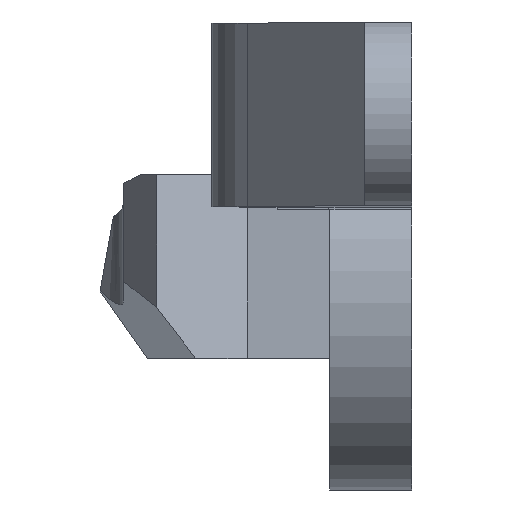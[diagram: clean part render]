
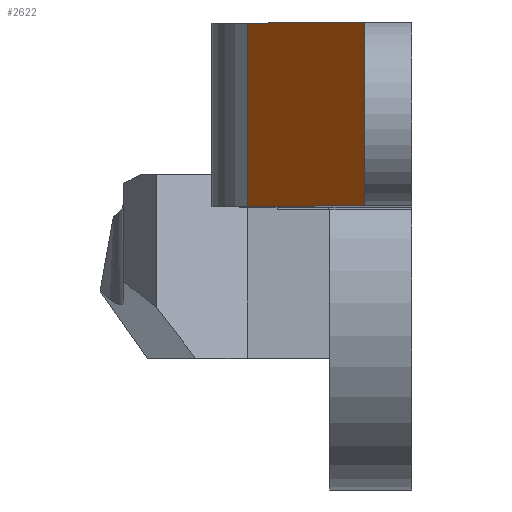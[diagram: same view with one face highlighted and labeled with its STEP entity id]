
A CAD part, top view. The second image highlights one B-rep face of the part: STEP entity #2622.
In plain terms, the highlighted planar face has unit normal (-0.985, 0, 0.174).
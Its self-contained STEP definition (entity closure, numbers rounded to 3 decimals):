
#1336 = PLANE('',#1337);
#1337 = AXIS2_PLACEMENT_3D('',#1338,#1339,#1340);
#1338 = CARTESIAN_POINT('',(-1.916,-1.752,-3.782));
#1339 = DIRECTION('',(0.,1.,0.));
#1340 = DIRECTION('',(0.,0.,1.));
#1388 = PLANE('',#1389);
#1389 = AXIS2_PLACEMENT_3D('',#1390,#1391,#1392);
#1390 = CARTESIAN_POINT('',(9.391,6.048,-3.639));
#1391 = DIRECTION('',(0.,1.,0.));
#1392 = DIRECTION('',(0.,0.,1.));
#2198 = VERTEX_POINT('',#2199);
#2199 = CARTESIAN_POINT('',(0.,6.048,
    -36.438));
#2212 = PLANE('',#2213);
#2213 = AXIS2_PLACEMENT_3D('',#2214,#2215,#2216);
#2214 = CARTESIAN_POINT('',(0.,0.,0.));
#2215 = DIRECTION('',(1.,0.,0.));
#2216 = DIRECTION('',(0.,0.,-1.));
#2223 = EDGE_CURVE('',#2198,#2224,#2226,.T.);
#2224 = VERTEX_POINT('',#2225);
#2225 = CARTESIAN_POINT('',(5.,6.048,-8.082));
#2226 = SURFACE_CURVE('',#2227,(#2231,#2237),.PCURVE_S1.);
#2227 = LINE('',#2228,#2229);
#2228 = CARTESIAN_POINT('',(6.062,6.048,
    -2.06));
#2229 = VECTOR('',#2230,1.);
#2230 = DIRECTION('',(0.174,0.,0.985
    ));
#2231 = PCURVE('',#1388,#2232);
#2232 = DEFINITIONAL_REPRESENTATION('',(#2233),#2236);
#2233 = B_SPLINE_CURVE_WITH_KNOTS('',1,(#2234,#2235),.UNSPECIFIED.,.F.,
  .F.,(2,2),(-37.788,-3.235),.PIECEWISE_BEZIER_KNOTS.);
#2234 = CARTESIAN_POINT('',(-35.635,-9.891));
#2235 = CARTESIAN_POINT('',(-1.608,-3.891));
#2236 = ( GEOMETRIC_REPRESENTATION_CONTEXT(2) 
PARAMETRIC_REPRESENTATION_CONTEXT() REPRESENTATION_CONTEXT('2D SPACE',''
  ) );
#2237 = PCURVE('',#2238,#2243);
#2238 = PLANE('',#2239);
#2239 = AXIS2_PLACEMENT_3D('',#2240,#2241,#2242);
#2240 = CARTESIAN_POINT('',(6.231,-38.298,
    -1.099));
#2241 = DIRECTION('',(0.985,0.,-0.174
    ));
#2242 = DIRECTION('',(-0.174,0.,
    -0.985));
#2243 = DEFINITIONAL_REPRESENTATION('',(#2244),#2247);
#2244 = B_SPLINE_CURVE_WITH_KNOTS('',1,(#2245,#2246),.UNSPECIFIED.,.F.,
  .F.,(2,2),(-37.788,-3.235),.PIECEWISE_BEZIER_KNOTS.);
#2245 = CARTESIAN_POINT('',(38.764,44.346));
#2246 = CARTESIAN_POINT('',(4.211,44.346));
#2247 = ( GEOMETRIC_REPRESENTATION_CONTEXT(2) 
PARAMETRIC_REPRESENTATION_CONTEXT() REPRESENTATION_CONTEXT('2D SPACE',''
  ) );
#2264 = PLANE('',#2265);
#2265 = AXIS2_PLACEMENT_3D('',#2266,#2267,#2268);
#2266 = CARTESIAN_POINT('',(5.,-38.298,0.));
#2267 = DIRECTION('',(-1.,0.,0.));
#2268 = DIRECTION('',(0.,0.,1.));
#2432 = VERTEX_POINT('',#2433);
#2433 = CARTESIAN_POINT('',(0.,-1.752,
    -36.438));
#2452 = EDGE_CURVE('',#2432,#2453,#2455,.T.);
#2453 = VERTEX_POINT('',#2454);
#2454 = CARTESIAN_POINT('',(5.,-1.752,-8.082));
#2455 = SURFACE_CURVE('',#2456,(#2460,#2466),.PCURVE_S1.);
#2456 = LINE('',#2457,#2458);
#2457 = CARTESIAN_POINT('',(5.879,-1.752,
    -3.096));
#2458 = VECTOR('',#2459,1.);
#2459 = DIRECTION('',(0.174,0.,0.985)
  );
#2460 = PCURVE('',#1336,#2461);
#2461 = DEFINITIONAL_REPRESENTATION('',(#2462),#2465);
#2462 = B_SPLINE_CURVE_WITH_KNOTS('',1,(#2463,#2464),.UNSPECIFIED.,.F.,
  .F.,(2,2),(-36.735,-2.183),.PIECEWISE_BEZIER_KNOTS.);
#2463 = CARTESIAN_POINT('',(-35.492,1.416));
#2464 = CARTESIAN_POINT('',(-1.464,7.416));
#2465 = ( GEOMETRIC_REPRESENTATION_CONTEXT(2) 
PARAMETRIC_REPRESENTATION_CONTEXT() REPRESENTATION_CONTEXT('2D SPACE',''
  ) );
#2466 = PCURVE('',#2238,#2467);
#2467 = DEFINITIONAL_REPRESENTATION('',(#2468),#2471);
#2468 = B_SPLINE_CURVE_WITH_KNOTS('',1,(#2469,#2470),.UNSPECIFIED.,.F.,
  .F.,(2,2),(-36.735,-2.183),.PIECEWISE_BEZIER_KNOTS.);
#2469 = CARTESIAN_POINT('',(38.764,36.546));
#2470 = CARTESIAN_POINT('',(4.211,36.546));
#2471 = ( GEOMETRIC_REPRESENTATION_CONTEXT(2) 
PARAMETRIC_REPRESENTATION_CONTEXT() REPRESENTATION_CONTEXT('2D SPACE',''
  ) );
#2599 = EDGE_CURVE('',#2453,#2224,#2600,.T.);
#2600 = SURFACE_CURVE('',#2601,(#2605,#2612),.PCURVE_S1.);
#2601 = LINE('',#2602,#2603);
#2602 = CARTESIAN_POINT('',(5.,-38.298,-8.082));
#2603 = VECTOR('',#2604,1.);
#2604 = DIRECTION('',(0.,1.,0.));
#2605 = PCURVE('',#2264,#2606);
#2606 = DEFINITIONAL_REPRESENTATION('',(#2607),#2611);
#2607 = LINE('',#2608,#2609);
#2608 = CARTESIAN_POINT('',(-8.082,0.));
#2609 = VECTOR('',#2610,1.);
#2610 = DIRECTION('',(0.,1.));
#2611 = ( GEOMETRIC_REPRESENTATION_CONTEXT(2) 
PARAMETRIC_REPRESENTATION_CONTEXT() REPRESENTATION_CONTEXT('2D SPACE',''
  ) );
#2612 = PCURVE('',#2238,#2613);
#2613 = DEFINITIONAL_REPRESENTATION('',(#2614),#2618);
#2614 = LINE('',#2615,#2616);
#2615 = CARTESIAN_POINT('',(7.091,0.));
#2616 = VECTOR('',#2617,1.);
#2617 = DIRECTION('',(0.,1.));
#2618 = ( GEOMETRIC_REPRESENTATION_CONTEXT(2) 
PARAMETRIC_REPRESENTATION_CONTEXT() REPRESENTATION_CONTEXT('2D SPACE',''
  ) );
#2622 = ADVANCED_FACE('',(#2623),#2238,.F.);
#2623 = FACE_BOUND('',#2624,.F.);
#2624 = EDGE_LOOP('',(#2625,#2626,#2647,#2648));
#2625 = ORIENTED_EDGE('',*,*,#2452,.F.);
#2626 = ORIENTED_EDGE('',*,*,#2627,.T.);
#2627 = EDGE_CURVE('',#2432,#2198,#2628,.T.);
#2628 = SURFACE_CURVE('',#2629,(#2633,#2640),.PCURVE_S1.);
#2629 = LINE('',#2630,#2631);
#2630 = CARTESIAN_POINT('',(0.,-38.298,
    -36.438));
#2631 = VECTOR('',#2632,1.);
#2632 = DIRECTION('',(0.,1.,0.));
#2633 = PCURVE('',#2238,#2634);
#2634 = DEFINITIONAL_REPRESENTATION('',(#2635),#2639);
#2635 = LINE('',#2636,#2637);
#2636 = CARTESIAN_POINT('',(35.885,0.));
#2637 = VECTOR('',#2638,1.);
#2638 = DIRECTION('',(0.,1.));
#2639 = ( GEOMETRIC_REPRESENTATION_CONTEXT(2) 
PARAMETRIC_REPRESENTATION_CONTEXT() REPRESENTATION_CONTEXT('2D SPACE',''
  ) );
#2640 = PCURVE('',#2212,#2641);
#2641 = DEFINITIONAL_REPRESENTATION('',(#2642),#2646);
#2642 = LINE('',#2643,#2644);
#2643 = CARTESIAN_POINT('',(36.438,-38.298));
#2644 = VECTOR('',#2645,1.);
#2645 = DIRECTION('',(0.,1.));
#2646 = ( GEOMETRIC_REPRESENTATION_CONTEXT(2) 
PARAMETRIC_REPRESENTATION_CONTEXT() REPRESENTATION_CONTEXT('2D SPACE',''
  ) );
#2647 = ORIENTED_EDGE('',*,*,#2223,.T.);
#2648 = ORIENTED_EDGE('',*,*,#2599,.F.);
